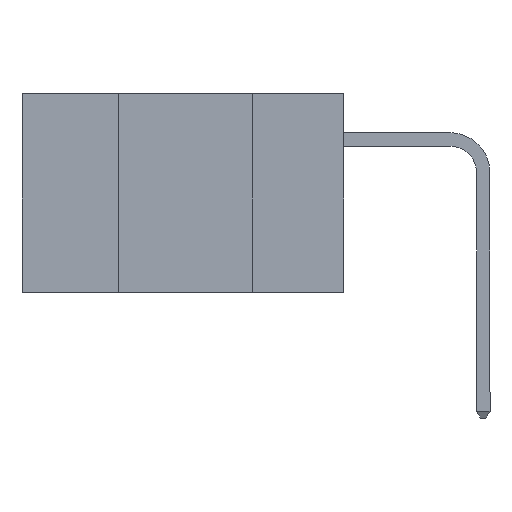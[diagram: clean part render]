
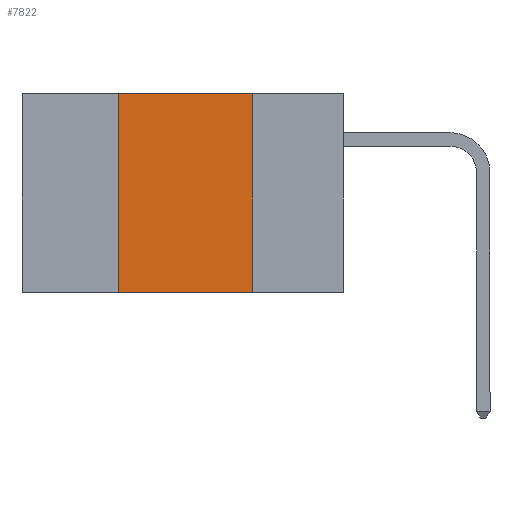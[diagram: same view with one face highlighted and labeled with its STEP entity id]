
A CAD part, left-side view. The second image highlights one B-rep face of the part: STEP entity #7822.
In plain terms, the highlighted planar face has unit normal (-1, 0, 0).
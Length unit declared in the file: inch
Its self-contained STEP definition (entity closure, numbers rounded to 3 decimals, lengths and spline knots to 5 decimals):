
#69 = LINE ( 'NONE', #10848, #5464 ) ;
#170 = ORIENTED_EDGE ( 'NONE', *, *, #11413, .F. ) ;
#648 = DIRECTION ( 'NONE',  ( 0., 0., -1. ) ) ;
#832 = ORIENTED_EDGE ( 'NONE', *, *, #9577, .T. ) ;
#922 = LINE ( 'NONE', #6201, #5913 ) ;
#1002 = CARTESIAN_POINT ( 'NONE',  ( 0., 0.42, 0. ) ) ;
#2168 = VECTOR ( 'NONE', #2834, 39.37008 ) ;
#2239 = DIRECTION ( 'NONE',  ( 0., -1., 0. ) ) ;
#2834 = DIRECTION ( 'NONE',  ( 0., -1., 0. ) ) ;
#3190 = CARTESIAN_POINT ( 'NONE',  ( 0., 0.42, -0.37 ) ) ;
#3211 = ORIENTED_EDGE ( 'NONE', *, *, #10961, .F. ) ;
#3340 = VERTEX_POINT ( 'NONE', #5663 ) ;
#4214 = LINE ( 'NONE', #8616, #2168 ) ;
#5275 = DIRECTION ( 'NONE',  ( 0., 0., 1. ) ) ;
#5342 = PLANE ( 'NONE',  #5692 ) ;
#5369 = VERTEX_POINT ( 'NONE', #6414 ) ;
#5464 = VECTOR ( 'NONE', #5275, 39.37008 ) ;
#5663 = CARTESIAN_POINT ( 'NONE',  ( 0., 0.17, -0.37 ) ) ;
#5692 = AXIS2_PLACEMENT_3D ( 'NONE', #11156, #7606, #7851 ) ;
#5802 = FACE_OUTER_BOUND ( 'NONE', #8034, .T. ) ;
#5913 = VECTOR ( 'NONE', #2239, 39.37008 ) ;
#6201 = CARTESIAN_POINT ( 'NONE',  ( 0., 0.6, -0.37 ) ) ;
#6414 = CARTESIAN_POINT ( 'NONE',  ( 0., 0.17, 0. ) ) ;
#7606 = DIRECTION ( 'NONE',  ( 1., 0., 0. ) ) ;
#7822 = ADVANCED_FACE ( 'NONE', ( #5802 ), #5342, .F. ) ;
#7851 = DIRECTION ( 'NONE',  ( 0., 0., -1. ) ) ;
#8034 = EDGE_LOOP ( 'NONE', ( #170, #3211, #8327, #832 ) ) ;
#8327 = ORIENTED_EDGE ( 'NONE', *, *, #10215, .F. ) ;
#8616 = CARTESIAN_POINT ( 'NONE',  ( 0., 0.6, 0. ) ) ;
#9577 = EDGE_CURVE ( 'NONE', #11157, #3340, #922, .T. ) ;
#10066 = VERTEX_POINT ( 'NONE', #1002 ) ;
#10215 = EDGE_CURVE ( 'NONE', #11157, #10066, #69, .T. ) ;
#10252 = LINE ( 'NONE', #12107, #12066 ) ;
#10848 = CARTESIAN_POINT ( 'NONE',  ( 0., 0.42, 0. ) ) ;
#10961 = EDGE_CURVE ( 'NONE', #10066, #5369, #4214, .T. ) ;
#11156 = CARTESIAN_POINT ( 'NONE',  ( 0., 0.6, 0. ) ) ;
#11157 = VERTEX_POINT ( 'NONE', #3190 ) ;
#11413 = EDGE_CURVE ( 'NONE', #5369, #3340, #10252, .T. ) ;
#12066 = VECTOR ( 'NONE', #648, 39.37008 ) ;
#12107 = CARTESIAN_POINT ( 'NONE',  ( 0., 0.17, 0. ) ) ;
